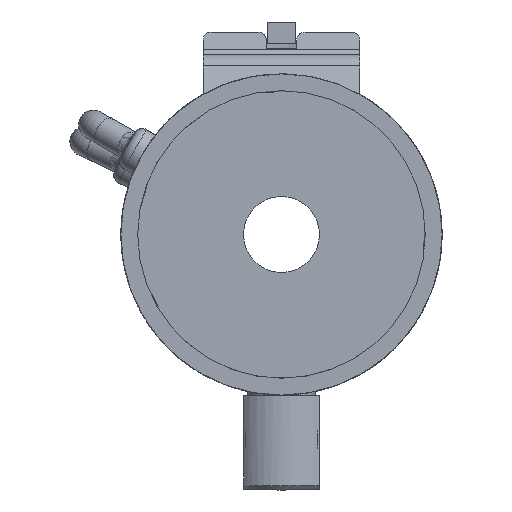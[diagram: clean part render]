
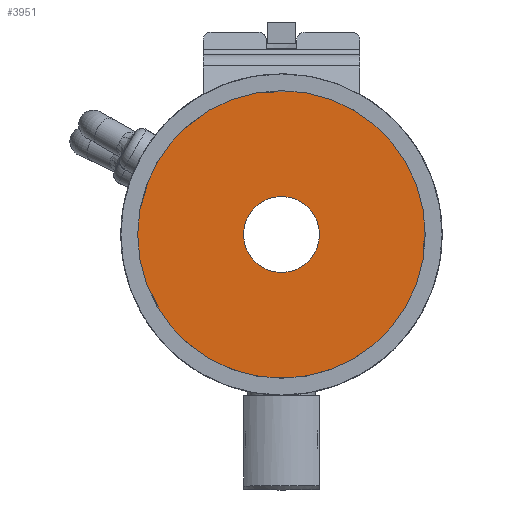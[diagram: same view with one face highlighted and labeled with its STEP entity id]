
A CAD part, front view. The second image highlights one B-rep face of the part: STEP entity #3951.
In plain terms, the highlighted planar face has unit normal (0, -1, 0).
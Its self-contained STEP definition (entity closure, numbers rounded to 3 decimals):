
#60=FACE_BOUND('',#618,.T.);
#192=PLANE('',#4284);
#370=FACE_OUTER_BOUND('',#617,.T.);
#617=EDGE_LOOP('',(#3433));
#618=EDGE_LOOP('',(#3434));
#765=CIRCLE('',#4187,4.5);
#796=CIRCLE('',#4285,17.05);
#1649=VERTEX_POINT('',#7639);
#1842=VERTEX_POINT('',#11338);
#2146=EDGE_CURVE('',#1649,#1649,#765,.T.);
#2401=EDGE_CURVE('',#1842,#1842,#796,.T.);
#3433=ORIENTED_EDGE('',*,*,#2401,.F.);
#3434=ORIENTED_EDGE('',*,*,#2146,.F.);
#3951=ADVANCED_FACE('',(#370,#60),#192,.F.);
#4187=AXIS2_PLACEMENT_3D('',#7641,#4752,#4753);
#4284=AXIS2_PLACEMENT_3D('',#11337,#5037,#5038);
#4285=AXIS2_PLACEMENT_3D('',#11339,#5039,#5040);
#4752=DIRECTION('center_axis',(0.,-1.,0.));
#4753=DIRECTION('ref_axis',(1.,0.,0.));
#5037=DIRECTION('center_axis',(0.,1.,0.));
#5038=DIRECTION('ref_axis',(1.,0.,0.));
#5039=DIRECTION('center_axis',(0.,1.,0.));
#5040=DIRECTION('ref_axis',(0.985,0.,-0.174));
#7639=CARTESIAN_POINT('',(545.5,919.647,-2132.196));
#7641=CARTESIAN_POINT('Origin',(550.,919.647,-2132.196));
#11337=CARTESIAN_POINT('Origin',(550.,919.647,-2132.196));
#11338=CARTESIAN_POINT('',(533.209,919.647,-2129.235));
#11339=CARTESIAN_POINT('Origin',(550.,919.647,-2132.196));
